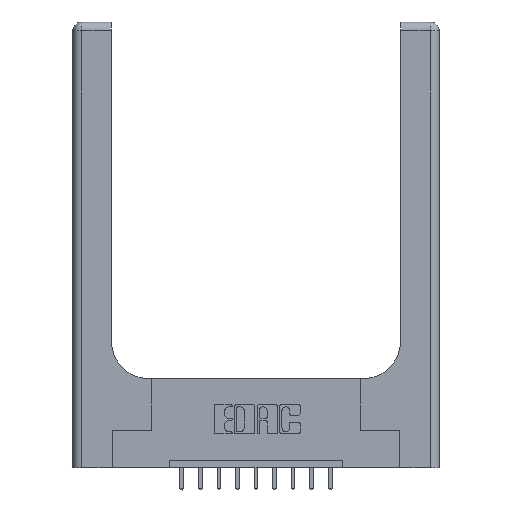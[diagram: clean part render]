
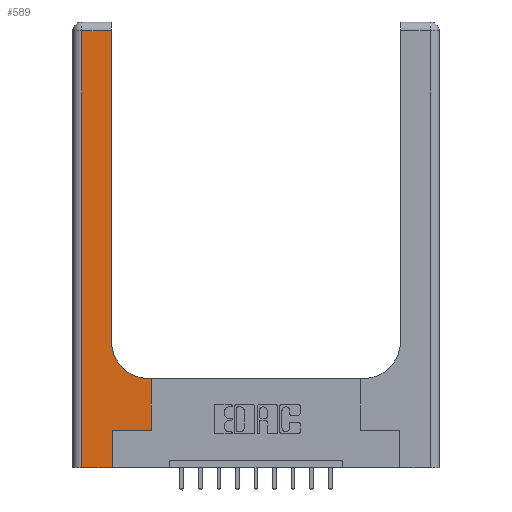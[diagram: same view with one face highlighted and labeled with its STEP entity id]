
A CAD part, top view. The second image highlights one B-rep face of the part: STEP entity #589.
In plain terms, the highlighted planar face has unit normal (0, 0, 1).
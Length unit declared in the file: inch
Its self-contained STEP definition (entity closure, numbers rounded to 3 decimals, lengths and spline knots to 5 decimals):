
#77 = CARTESIAN_POINT ( 'NONE',  ( 0.265, 0., 0.37 ) ) ;
#333 = LINE ( 'NONE', #6307, #1952 ) ;
#513 = LINE ( 'NONE', #8992, #3065 ) ;
#572 = VERTEX_POINT ( 'NONE', #2977 ) ;
#589 = ADVANCED_FACE ( 'NONE', ( #4679 ), #5790, .F. ) ;
#683 = CARTESIAN_POINT ( 'NONE',  ( 0.26, 0.6, 0.37 ) ) ;
#1038 = VERTEX_POINT ( 'NONE', #13701 ) ;
#1067 = DIRECTION ( 'NONE',  ( 1., 0., 0. ) ) ;
#1201 = DIRECTION ( 'NONE',  ( 0., 1., 0. ) ) ;
#1453 = LINE ( 'NONE', #10482, #6438 ) ;
#1919 = DIRECTION ( 'NONE',  ( 0., -1., 0. ) ) ;
#1952 = VECTOR ( 'NONE', #4241, 39.37008 ) ;
#2020 = CARTESIAN_POINT ( 'NONE',  ( 0.528, 0.25, 0.37 ) ) ;
#2148 = ORIENTED_EDGE ( 'NONE', *, *, #9514, .T. ) ;
#2209 = CARTESIAN_POINT ( 'NONE',  ( 0.528, 0.25, 0.37 ) ) ;
#2270 = EDGE_CURVE ( 'NONE', #12200, #12806, #3889, .T. ) ;
#2379 = DIRECTION ( 'NONE',  ( 1., 0., 0. ) ) ;
#2482 = ORIENTED_EDGE ( 'NONE', *, *, #13859, .T. ) ;
#2499 = DIRECTION ( 'NONE',  ( 0., 1., 0. ) ) ;
#2847 = CARTESIAN_POINT ( 'NONE',  ( 0.06, 0., 0.37 ) ) ;
#2977 = CARTESIAN_POINT ( 'NONE',  ( 0.06, 2.94, 0.37 ) ) ;
#3065 = VECTOR ( 'NONE', #1919, 39.37008 ) ;
#3777 = DIRECTION ( 'NONE',  ( 0., 1., 0. ) ) ;
#3889 = LINE ( 'NONE', #77, #7957 ) ;
#4241 = DIRECTION ( 'NONE',  ( -1., 0., 0. ) ) ;
#4420 = EDGE_CURVE ( 'NONE', #1038, #572, #333, .T. ) ;
#4679 = FACE_OUTER_BOUND ( 'NONE', #13130, .T. ) ;
#4955 = CARTESIAN_POINT ( 'NONE',  ( 0.265, 0., 0.37 ) ) ;
#5080 = VERTEX_POINT ( 'NONE', #7888 ) ;
#5157 = ORIENTED_EDGE ( 'NONE', *, *, #12007, .T. ) ;
#5191 = VECTOR ( 'NONE', #1201, 39.37008 ) ;
#5497 = ORIENTED_EDGE ( 'NONE', *, *, #12763, .T. ) ;
#5577 = CARTESIAN_POINT ( 'NONE',  ( 0., 3., 0.37 ) ) ;
#5790 = PLANE ( 'NONE',  #7021 ) ;
#5873 = CARTESIAN_POINT ( 'NONE',  ( 0.26, 3., 0.37 ) ) ;
#6034 = CARTESIAN_POINT ( 'NONE',  ( 0.26, 0.85, 0.37 ) ) ;
#6307 = CARTESIAN_POINT ( 'NONE',  ( 0., 2.94, 0.37 ) ) ;
#6379 = VECTOR ( 'NONE', #6498, 39.37008 ) ;
#6438 = VECTOR ( 'NONE', #11670, 39.37008 ) ;
#6498 = DIRECTION ( 'NONE',  ( -1., 0., 0. ) ) ;
#6802 = EDGE_CURVE ( 'NONE', #12547, #7614, #8354, .T. ) ;
#7021 = AXIS2_PLACEMENT_3D ( 'NONE', #5577, #9175, #15080 ) ;
#7169 = VECTOR ( 'NONE', #2379, 39.37008 ) ;
#7614 = VERTEX_POINT ( 'NONE', #6034 ) ;
#7888 = CARTESIAN_POINT ( 'NONE',  ( 0.528, 0.6, 0.37 ) ) ;
#7957 = VECTOR ( 'NONE', #3777, 39.37008 ) ;
#8025 = ORIENTED_EDGE ( 'NONE', *, *, #6802, .T. ) ;
#8217 = DIRECTION ( 'NONE',  ( 0., 0., -1. ) ) ;
#8316 = CARTESIAN_POINT ( 'NONE',  ( 0.265, 0.25, 0.37 ) ) ;
#8354 = CIRCLE ( 'NONE', #14571, 0.25 ) ;
#8835 = LINE ( 'NONE', #5873, #9788 ) ;
#8992 = CARTESIAN_POINT ( 'NONE',  ( 0.06, 3., 0.37 ) ) ;
#9175 = DIRECTION ( 'NONE',  ( 0., 0., -1. ) ) ;
#9514 = EDGE_CURVE ( 'NONE', #5080, #12547, #14465, .T. ) ;
#9615 = ORIENTED_EDGE ( 'NONE', *, *, #2270, .T. ) ;
#9788 = VECTOR ( 'NONE', #2499, 39.37008 ) ;
#10482 = CARTESIAN_POINT ( 'NONE',  ( 0., 0., 0.37 ) ) ;
#10737 = LINE ( 'NONE', #2209, #5191 ) ;
#11199 = VERTEX_POINT ( 'NONE', #2020 ) ;
#11670 = DIRECTION ( 'NONE',  ( 1., 0., 0. ) ) ;
#11746 = CARTESIAN_POINT ( 'NONE',  ( 0.265, 0.25, 0.37 ) ) ;
#12007 = EDGE_CURVE ( 'NONE', #11199, #5080, #10737, .T. ) ;
#12200 = VERTEX_POINT ( 'NONE', #4955 ) ;
#12547 = VERTEX_POINT ( 'NONE', #15111 ) ;
#12597 = ORIENTED_EDGE ( 'NONE', *, *, #13723, .T. ) ;
#12763 = EDGE_CURVE ( 'NONE', #7614, #1038, #8835, .T. ) ;
#12806 = VERTEX_POINT ( 'NONE', #11746 ) ;
#12943 = VERTEX_POINT ( 'NONE', #2847 ) ;
#13072 = ORIENTED_EDGE ( 'NONE', *, *, #4420, .T. ) ;
#13130 = EDGE_LOOP ( 'NONE', ( #5497, #13072, #13385, #12597, #9615, #2482, #5157, #2148, #8025 ) ) ;
#13385 = ORIENTED_EDGE ( 'NONE', *, *, #14850, .T. ) ;
#13701 = CARTESIAN_POINT ( 'NONE',  ( 0.26, 2.94, 0.37 ) ) ;
#13723 = EDGE_CURVE ( 'NONE', #12943, #12200, #1453, .T. ) ;
#13859 = EDGE_CURVE ( 'NONE', #12806, #11199, #15053, .T. ) ;
#14465 = LINE ( 'NONE', #683, #6379 ) ;
#14571 = AXIS2_PLACEMENT_3D ( 'NONE', #15149, #8217, #1067 ) ;
#14850 = EDGE_CURVE ( 'NONE', #572, #12943, #513, .T. ) ;
#15053 = LINE ( 'NONE', #8316, #7169 ) ;
#15080 = DIRECTION ( 'NONE',  ( -1., 0., 0. ) ) ;
#15111 = CARTESIAN_POINT ( 'NONE',  ( 0.51, 0.6, 0.37 ) ) ;
#15149 = CARTESIAN_POINT ( 'NONE',  ( 0.51, 0.85, 0.37 ) ) ;
